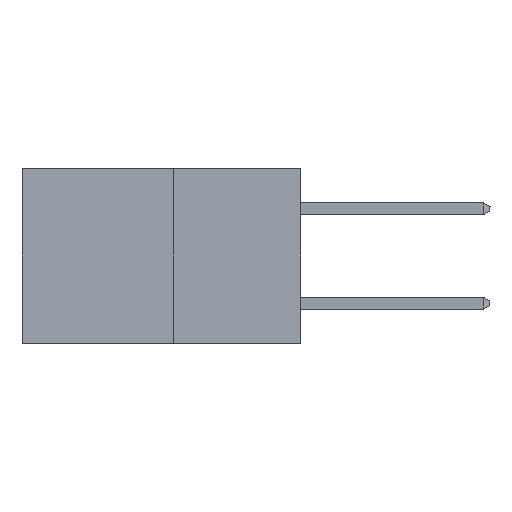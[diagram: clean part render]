
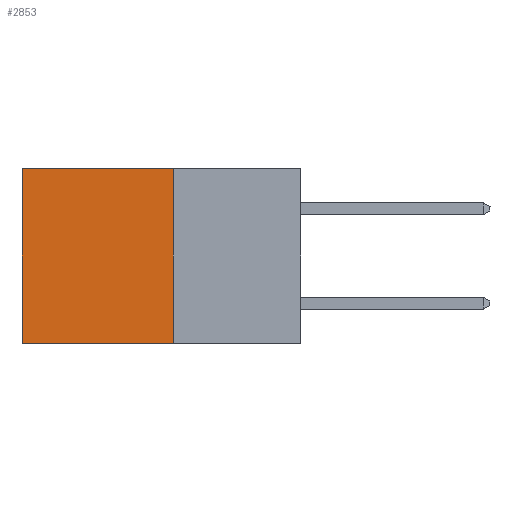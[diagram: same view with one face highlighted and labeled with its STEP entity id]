
A CAD part, left-side view. The second image highlights one B-rep face of the part: STEP entity #2853.
In plain terms, the highlighted planar face has unit normal (-1, 0, 0).
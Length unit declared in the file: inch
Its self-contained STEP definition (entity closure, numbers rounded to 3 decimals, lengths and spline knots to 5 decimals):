
#896 = ORIENTED_EDGE ( 'NONE', *, *, #12376, .F. ) ;
#1258 = ORIENTED_EDGE ( 'NONE', *, *, #3382, .T. ) ;
#1279 = FACE_OUTER_BOUND ( 'NONE', #4949, .T. ) ;
#2173 = EDGE_CURVE ( 'NONE', #6395, #5160, #10085, .T. ) ;
#2853 = ADVANCED_FACE ( 'NONE', ( #1279 ), #5134, .F. ) ;
#3382 = EDGE_CURVE ( 'NONE', #9168, #9166, #11689, .T. ) ;
#3987 = DIRECTION ( 'NONE',  ( 0., 0., -1. ) ) ;
#4070 = DIRECTION ( 'NONE',  ( 1., 0., 0. ) ) ;
#4270 = VECTOR ( 'NONE', #7072, 39.37008 ) ;
#4421 = CARTESIAN_POINT ( 'NONE',  ( 0.277, 0.27, -0.37 ) ) ;
#4623 = LINE ( 'NONE', #13885, #11747 ) ;
#4719 = LINE ( 'NONE', #12389, #7695 ) ;
#4949 = EDGE_LOOP ( 'NONE', ( #10043, #12325, #896, #1258 ) ) ;
#5134 = PLANE ( 'NONE',  #11198 ) ;
#5160 = VERTEX_POINT ( 'NONE', #8945 ) ;
#5969 = DIRECTION ( 'NONE',  ( 0., 0., -1. ) ) ;
#6021 = CARTESIAN_POINT ( 'NONE',  ( 0.277, 0.27, 0. ) ) ;
#6395 = VERTEX_POINT ( 'NONE', #8372 ) ;
#6995 = CARTESIAN_POINT ( 'NONE',  ( 0.277, 0.27, -0.37 ) ) ;
#7072 = DIRECTION ( 'NONE',  ( 0., 1., 0. ) ) ;
#7695 = VECTOR ( 'NONE', #5969, 39.37008 ) ;
#8372 = CARTESIAN_POINT ( 'NONE',  ( 0.277, 0.27, -0.37 ) ) ;
#8645 = DIRECTION ( 'NONE',  ( 0., 0., -1. ) ) ;
#8945 = CARTESIAN_POINT ( 'NONE',  ( 0.277, 0.59, -0.37 ) ) ;
#9129 = EDGE_CURVE ( 'NONE', #9166, #5160, #4719, .T. ) ;
#9166 = VERTEX_POINT ( 'NONE', #12430 ) ;
#9168 = VERTEX_POINT ( 'NONE', #6021 ) ;
#10043 = ORIENTED_EDGE ( 'NONE', *, *, #9129, .T. ) ;
#10085 = LINE ( 'NONE', #6995, #4270 ) ;
#10607 = CARTESIAN_POINT ( 'NONE',  ( 0.277, 0.27, 0. ) ) ;
#10706 = DIRECTION ( 'NONE',  ( 0., 1., 0. ) ) ;
#11198 = AXIS2_PLACEMENT_3D ( 'NONE', #4421, #4070, #3987 ) ;
#11358 = VECTOR ( 'NONE', #10706, 39.37008 ) ;
#11689 = LINE ( 'NONE', #10607, #11358 ) ;
#11747 = VECTOR ( 'NONE', #8645, 39.37008 ) ;
#12325 = ORIENTED_EDGE ( 'NONE', *, *, #2173, .F. ) ;
#12376 = EDGE_CURVE ( 'NONE', #9168, #6395, #4623, .T. ) ;
#12389 = CARTESIAN_POINT ( 'NONE',  ( 0.277, 0.59, -0.37 ) ) ;
#12430 = CARTESIAN_POINT ( 'NONE',  ( 0.277, 0.59, 0. ) ) ;
#13885 = CARTESIAN_POINT ( 'NONE',  ( 0.277, 0.27, -0.37 ) ) ;
